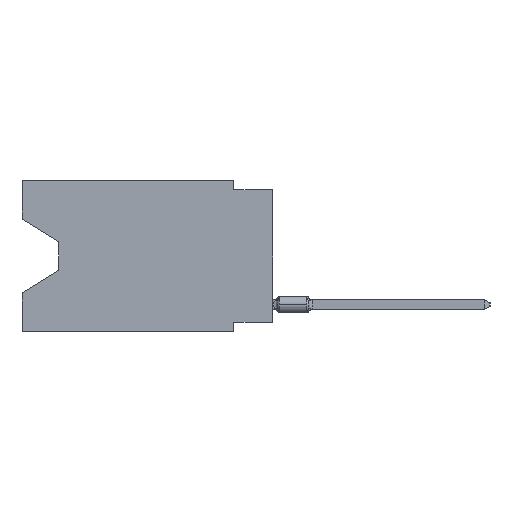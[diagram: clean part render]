
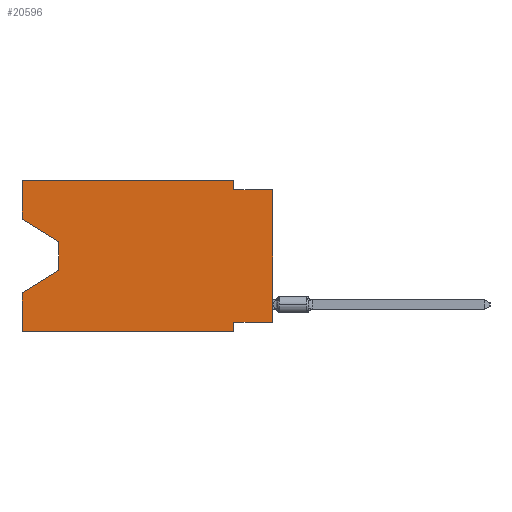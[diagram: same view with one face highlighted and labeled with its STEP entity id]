
A CAD part, left-side view. The second image highlights one B-rep face of the part: STEP entity #20596.
In plain terms, the highlighted planar face has unit normal (-1, 0, 0).
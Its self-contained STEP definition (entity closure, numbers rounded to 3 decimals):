
#254 = VERTEX_POINT ( 'NONE', #10600 ) ;
#603 = ORIENTED_EDGE ( 'NONE', *, *, #19769, .T. ) ;
#863 = CARTESIAN_POINT ( 'NONE',  ( 0., 16.383, -9.906 ) ) ;
#980 = DIRECTION ( 'NONE',  ( 0., 0.855, -0.519 ) ) ;
#1502 = CARTESIAN_POINT ( 'NONE',  ( 0., 13.97, -5.893 ) ) ;
#2517 = LINE ( 'NONE', #7267, #28062 ) ;
#2779 = VERTEX_POINT ( 'NONE', #863 ) ;
#2851 = DIRECTION ( 'NONE',  ( 0., 0., -1. ) ) ;
#2890 = VECTOR ( 'NONE', #24371, 1000. ) ;
#4055 = CARTESIAN_POINT ( 'NONE',  ( 0., 0., 0. ) ) ;
#4206 = LINE ( 'NONE', #26165, #24664 ) ;
#5468 = CARTESIAN_POINT ( 'NONE',  ( 0., 0., -9.271 ) ) ;
#5710 = ORIENTED_EDGE ( 'NONE', *, *, #22553, .T. ) ;
#6392 = ORIENTED_EDGE ( 'NONE', *, *, #29859, .F. ) ;
#6566 = VECTOR ( 'NONE', #20122, 1000. ) ;
#6790 = DIRECTION ( 'NONE',  ( 0., 0., 1. ) ) ;
#7185 = DIRECTION ( 'NONE',  ( 0., 0., -1. ) ) ;
#7267 = CARTESIAN_POINT ( 'NONE',  ( 0., 0., -0.635 ) ) ;
#7303 = LINE ( 'NONE', #28563, #20341 ) ;
#7872 = CARTESIAN_POINT ( 'NONE',  ( 0., 2.54, -9.271 ) ) ;
#9094 = EDGE_CURVE ( 'NONE', #12680, #22401, #18404, .T. ) ;
#9250 = ORIENTED_EDGE ( 'NONE', *, *, #15418, .T. ) ;
#9877 = CARTESIAN_POINT ( 'NONE',  ( 0., 16.383, -2.546 ) ) ;
#10276 = VERTEX_POINT ( 'NONE', #7872 ) ;
#10499 = CARTESIAN_POINT ( 'NONE',  ( 0., 13.97, -5.893 ) ) ;
#10600 = CARTESIAN_POINT ( 'NONE',  ( 0., 16.383, 0. ) ) ;
#11370 = EDGE_CURVE ( 'NONE', #13501, #11434, #4206, .T. ) ;
#11434 = VERTEX_POINT ( 'NONE', #10499 ) ;
#11438 = CARTESIAN_POINT ( 'NONE',  ( 0., 16.383, 0. ) ) ;
#11549 = CARTESIAN_POINT ( 'NONE',  ( 0., 13.97, -4.013 ) ) ;
#12680 = VERTEX_POINT ( 'NONE', #5468 ) ;
#12792 = LINE ( 'NONE', #20900, #22035 ) ;
#13002 = CARTESIAN_POINT ( 'NONE',  ( 0., 2.54, -0.635 ) ) ;
#13501 = VERTEX_POINT ( 'NONE', #11549 ) ;
#14766 = DIRECTION ( 'NONE',  ( 0., 0., 1. ) ) ;
#15006 = DIRECTION ( 'NONE',  ( 0., 1., 0. ) ) ;
#15418 = EDGE_CURVE ( 'NONE', #11434, #25249, #20113, .T. ) ;
#15549 = EDGE_CURVE ( 'NONE', #12680, #10276, #23117, .T. ) ;
#15729 = ORIENTED_EDGE ( 'NONE', *, *, #9094, .T. ) ;
#16687 = ORIENTED_EDGE ( 'NONE', *, *, #33347, .F. ) ;
#17315 = LINE ( 'NONE', #33296, #6566 ) ;
#17430 = VECTOR ( 'NONE', #980, 1000. ) ;
#17703 = VERTEX_POINT ( 'NONE', #13002 ) ;
#18404 = LINE ( 'NONE', #4055, #26218 ) ;
#18515 = DIRECTION ( 'NONE',  ( 0., 0., -1. ) ) ;
#19563 = ORIENTED_EDGE ( 'NONE', *, *, #29012, .F. ) ;
#19769 = EDGE_CURVE ( 'NONE', #2779, #23295, #34597, .T. ) ;
#20113 = LINE ( 'NONE', #1502, #17430 ) ;
#20116 = VECTOR ( 'NONE', #32661, 1000. ) ;
#20122 = DIRECTION ( 'NONE',  ( 0., 0., 1. ) ) ;
#20341 = VECTOR ( 'NONE', #6790, 1000. ) ;
#20379 = DIRECTION ( 'NONE',  ( 0., -1., 0. ) ) ;
#20527 = VECTOR ( 'NONE', #33940, 1000. ) ;
#20596 = ADVANCED_FACE ( 'NONE', ( #29545 ), #32189, .F. ) ;
#20900 = CARTESIAN_POINT ( 'NONE',  ( 0., 16.383, 0. ) ) ;
#20949 = VERTEX_POINT ( 'NONE', #31465 ) ;
#21013 = ORIENTED_EDGE ( 'NONE', *, *, #15549, .F. ) ;
#21557 = LINE ( 'NONE', #27002, #2890 ) ;
#22002 = DIRECTION ( 'NONE',  ( 1., 0., 0. ) ) ;
#22035 = VECTOR ( 'NONE', #20379, 1000. ) ;
#22184 = EDGE_CURVE ( 'NONE', #20949, #17703, #24312, .T. ) ;
#22401 = VERTEX_POINT ( 'NONE', #27118 ) ;
#22553 = EDGE_CURVE ( 'NONE', #25266, #13501, #34112, .T. ) ;
#23117 = LINE ( 'NONE', #31001, #34290 ) ;
#23295 = VERTEX_POINT ( 'NONE', #25186 ) ;
#24076 = CARTESIAN_POINT ( 'NONE',  ( 0., 16.383, -9.906 ) ) ;
#24312 = LINE ( 'NONE', #29054, #26149 ) ;
#24371 = DIRECTION ( 'NONE',  ( 0., 0., -1. ) ) ;
#24664 = VECTOR ( 'NONE', #7185, 1000. ) ;
#25027 = ORIENTED_EDGE ( 'NONE', *, *, #33048, .F. ) ;
#25139 = AXIS2_PLACEMENT_3D ( 'NONE', #11438, #22002, #2851 ) ;
#25186 = CARTESIAN_POINT ( 'NONE',  ( 0., 2.54, -9.906 ) ) ;
#25249 = VERTEX_POINT ( 'NONE', #26480 ) ;
#25266 = VERTEX_POINT ( 'NONE', #32243 ) ;
#25940 = ORIENTED_EDGE ( 'NONE', *, *, #26835, .F. ) ;
#26149 = VECTOR ( 'NONE', #18515, 1000. ) ;
#26165 = CARTESIAN_POINT ( 'NONE',  ( 0., 13.97, -4.013 ) ) ;
#26218 = VECTOR ( 'NONE', #14766, 1000. ) ;
#26480 = CARTESIAN_POINT ( 'NONE',  ( 0., 16.383, -7.36 ) ) ;
#26747 = EDGE_LOOP ( 'NONE', ( #5710, #30427, #9250, #16687, #603, #25027, #21013, #15729, #19563, #31826, #6392, #25940 ) ) ;
#26835 = EDGE_CURVE ( 'NONE', #25266, #254, #17315, .T. ) ;
#27002 = CARTESIAN_POINT ( 'NONE',  ( 0., 2.54, -9.906 ) ) ;
#27118 = CARTESIAN_POINT ( 'NONE',  ( 0., 0., -0.635 ) ) ;
#28062 = VECTOR ( 'NONE', #31680, 1000. ) ;
#28563 = CARTESIAN_POINT ( 'NONE',  ( 0., 16.383, 0. ) ) ;
#29012 = EDGE_CURVE ( 'NONE', #17703, #22401, #2517, .T. ) ;
#29054 = CARTESIAN_POINT ( 'NONE',  ( 0., 2.54, 0. ) ) ;
#29545 = FACE_OUTER_BOUND ( 'NONE', #26747, .T. ) ;
#29859 = EDGE_CURVE ( 'NONE', #254, #20949, #12792, .T. ) ;
#30427 = ORIENTED_EDGE ( 'NONE', *, *, #11370, .T. ) ;
#31001 = CARTESIAN_POINT ( 'NONE',  ( 0., 0., -9.271 ) ) ;
#31465 = CARTESIAN_POINT ( 'NONE',  ( 0., 2.54, 0. ) ) ;
#31680 = DIRECTION ( 'NONE',  ( 0., -1., 0. ) ) ;
#31826 = ORIENTED_EDGE ( 'NONE', *, *, #22184, .F. ) ;
#32189 = PLANE ( 'NONE',  #25139 ) ;
#32243 = CARTESIAN_POINT ( 'NONE',  ( 0., 16.383, -2.546 ) ) ;
#32661 = DIRECTION ( 'NONE',  ( 0., -1., 0. ) ) ;
#33048 = EDGE_CURVE ( 'NONE', #10276, #23295, #21557, .T. ) ;
#33296 = CARTESIAN_POINT ( 'NONE',  ( 0., 16.383, 0. ) ) ;
#33347 = EDGE_CURVE ( 'NONE', #2779, #25249, #7303, .T. ) ;
#33940 = DIRECTION ( 'NONE',  ( 0., -0.855, -0.519 ) ) ;
#34112 = LINE ( 'NONE', #9877, #20527 ) ;
#34290 = VECTOR ( 'NONE', #15006, 1000. ) ;
#34597 = LINE ( 'NONE', #24076, #20116 ) ;
